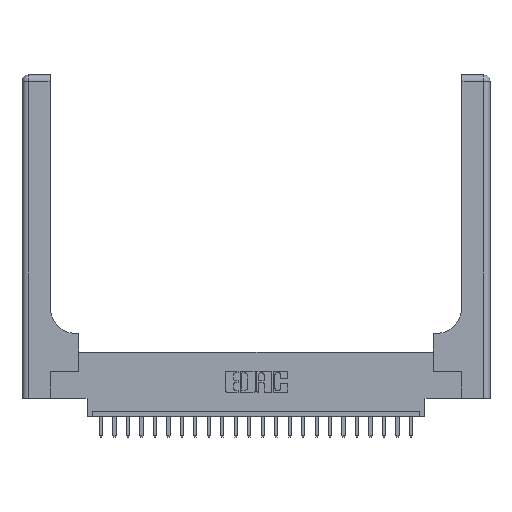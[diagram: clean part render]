
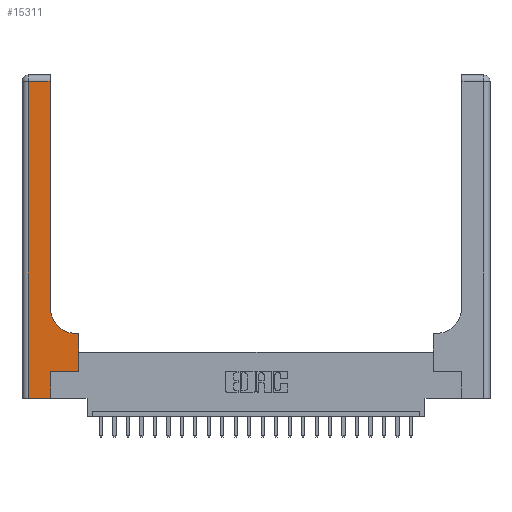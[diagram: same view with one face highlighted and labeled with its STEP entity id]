
A CAD part, top view. The second image highlights one B-rep face of the part: STEP entity #15311.
In plain terms, the highlighted planar face has unit normal (0, 0, 1).
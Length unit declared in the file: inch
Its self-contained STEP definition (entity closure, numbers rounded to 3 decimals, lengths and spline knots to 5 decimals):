
#444 = EDGE_CURVE ( 'NONE', #4858, #15761, #22272, .T. ) ;
#797 = ORIENTED_EDGE ( 'NONE', *, *, #22065, .T. ) ;
#800 = EDGE_LOOP ( 'NONE', ( #10502, #19393, #2431, #15078, #16799, #797, #15672, #21341, #15324 ) ) ;
#873 = CARTESIAN_POINT ( 'NONE',  ( 0., 3., 0.37 ) ) ;
#1178 = VECTOR ( 'NONE', #7933, 39.37008 ) ;
#1437 = DIRECTION ( 'NONE',  ( 0., 0., -1. ) ) ;
#2431 = ORIENTED_EDGE ( 'NONE', *, *, #10443, .T. ) ;
#2660 = LINE ( 'NONE', #7827, #13145 ) ;
#3457 = EDGE_CURVE ( 'NONE', #10535, #11096, #20568, .T. ) ;
#4597 = DIRECTION ( 'NONE',  ( 0., 1., 0. ) ) ;
#4659 = LINE ( 'NONE', #15798, #20899 ) ;
#4728 = EDGE_CURVE ( 'NONE', #7621, #4858, #4659, .T. ) ;
#4858 = VERTEX_POINT ( 'NONE', #7353 ) ;
#4860 = CARTESIAN_POINT ( 'NONE',  ( 0.06, 0., 0.37 ) ) ;
#5445 = DIRECTION ( 'NONE',  ( 0., 1., 0. ) ) ;
#6035 = CARTESIAN_POINT ( 'NONE',  ( 0.26, 0.85, 0.37 ) ) ;
#6046 = CARTESIAN_POINT ( 'NONE',  ( 0.265, 0.25, 0.37 ) ) ;
#6417 = CARTESIAN_POINT ( 'NONE',  ( 0., 2.94, 0.37 ) ) ;
#7353 = CARTESIAN_POINT ( 'NONE',  ( 0.26, 2.94, 0.37 ) ) ;
#7540 = EDGE_CURVE ( 'NONE', #14617, #7621, #7830, .T. ) ;
#7621 = VERTEX_POINT ( 'NONE', #6035 ) ;
#7814 = LINE ( 'NONE', #6046, #1178 ) ;
#7827 = CARTESIAN_POINT ( 'NONE',  ( 0.06, 3., 0.37 ) ) ;
#7830 = CIRCLE ( 'NONE', #9337, 0.25 ) ;
#7933 = DIRECTION ( 'NONE',  ( 1., 0., 0. ) ) ;
#9243 = VECTOR ( 'NONE', #16653, 39.37008 ) ;
#9337 = AXIS2_PLACEMENT_3D ( 'NONE', #19260, #1437, #22895 ) ;
#9482 = DIRECTION ( 'NONE',  ( -1., 0., 0. ) ) ;
#9760 = VECTOR ( 'NONE', #9482, 39.37008 ) ;
#9777 = PLANE ( 'NONE',  #10656 ) ;
#10443 = EDGE_CURVE ( 'NONE', #15761, #20156, #2660, .T. ) ;
#10502 = ORIENTED_EDGE ( 'NONE', *, *, #4728, .T. ) ;
#10535 = VERTEX_POINT ( 'NONE', #12159 ) ;
#10656 = AXIS2_PLACEMENT_3D ( 'NONE', #873, #16930, #17272 ) ;
#11096 = VERTEX_POINT ( 'NONE', #21508 ) ;
#11307 = EDGE_CURVE ( 'NONE', #14319, #15223, #17141, .T. ) ;
#11531 = FACE_OUTER_BOUND ( 'NONE', #800, .T. ) ;
#12159 = CARTESIAN_POINT ( 'NONE',  ( 0.528, 0.25, 0.37 ) ) ;
#12761 = CARTESIAN_POINT ( 'NONE',  ( 0.06, 2.94, 0.37 ) ) ;
#13001 = LINE ( 'NONE', #13335, #9760 ) ;
#13145 = VECTOR ( 'NONE', #18599, 39.37008 ) ;
#13335 = CARTESIAN_POINT ( 'NONE',  ( 0.26, 0.6, 0.37 ) ) ;
#13468 = CARTESIAN_POINT ( 'NONE',  ( 0., 0., 0.37 ) ) ;
#13576 = DIRECTION ( 'NONE',  ( -1., 0., 0. ) ) ;
#14032 = DIRECTION ( 'NONE',  ( 0., 1., 0. ) ) ;
#14319 = VERTEX_POINT ( 'NONE', #22391 ) ;
#14617 = VERTEX_POINT ( 'NONE', #18260 ) ;
#15078 = ORIENTED_EDGE ( 'NONE', *, *, #18080, .T. ) ;
#15223 = VERTEX_POINT ( 'NONE', #22570 ) ;
#15311 = ADVANCED_FACE ( 'NONE', ( #11531 ), #9777, .F. ) ;
#15324 = ORIENTED_EDGE ( 'NONE', *, *, #7540, .T. ) ;
#15672 = ORIENTED_EDGE ( 'NONE', *, *, #3457, .T. ) ;
#15761 = VERTEX_POINT ( 'NONE', #12761 ) ;
#15798 = CARTESIAN_POINT ( 'NONE',  ( 0.26, 3., 0.37 ) ) ;
#16653 = DIRECTION ( 'NONE',  ( 1., 0., 0. ) ) ;
#16799 = ORIENTED_EDGE ( 'NONE', *, *, #11307, .T. ) ;
#16896 = VECTOR ( 'NONE', #13576, 39.37008 ) ;
#16930 = DIRECTION ( 'NONE',  ( 0., 0., -1. ) ) ;
#17141 = LINE ( 'NONE', #17488, #21815 ) ;
#17272 = DIRECTION ( 'NONE',  ( -1., 0., 0. ) ) ;
#17488 = CARTESIAN_POINT ( 'NONE',  ( 0.265, 0., 0.37 ) ) ;
#17519 = CARTESIAN_POINT ( 'NONE',  ( 0.528, 0.25, 0.37 ) ) ;
#18080 = EDGE_CURVE ( 'NONE', #20156, #14319, #18288, .T. ) ;
#18260 = CARTESIAN_POINT ( 'NONE',  ( 0.51, 0.6, 0.37 ) ) ;
#18288 = LINE ( 'NONE', #13468, #9243 ) ;
#18599 = DIRECTION ( 'NONE',  ( 0., -1., 0. ) ) ;
#19169 = VECTOR ( 'NONE', #5445, 39.37008 ) ;
#19260 = CARTESIAN_POINT ( 'NONE',  ( 0.51, 0.85, 0.37 ) ) ;
#19393 = ORIENTED_EDGE ( 'NONE', *, *, #444, .T. ) ;
#19572 = EDGE_CURVE ( 'NONE', #11096, #14617, #13001, .T. ) ;
#20156 = VERTEX_POINT ( 'NONE', #4860 ) ;
#20568 = LINE ( 'NONE', #17519, #19169 ) ;
#20899 = VECTOR ( 'NONE', #14032, 39.37008 ) ;
#21341 = ORIENTED_EDGE ( 'NONE', *, *, #19572, .T. ) ;
#21508 = CARTESIAN_POINT ( 'NONE',  ( 0.528, 0.6, 0.37 ) ) ;
#21815 = VECTOR ( 'NONE', #4597, 39.37008 ) ;
#22065 = EDGE_CURVE ( 'NONE', #15223, #10535, #7814, .T. ) ;
#22272 = LINE ( 'NONE', #6417, #16896 ) ;
#22391 = CARTESIAN_POINT ( 'NONE',  ( 0.265, 0., 0.37 ) ) ;
#22570 = CARTESIAN_POINT ( 'NONE',  ( 0.265, 0.25, 0.37 ) ) ;
#22895 = DIRECTION ( 'NONE',  ( 1., 0., 0. ) ) ;
